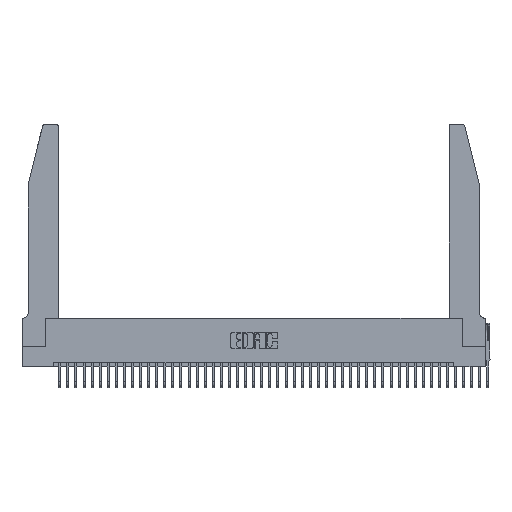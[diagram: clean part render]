
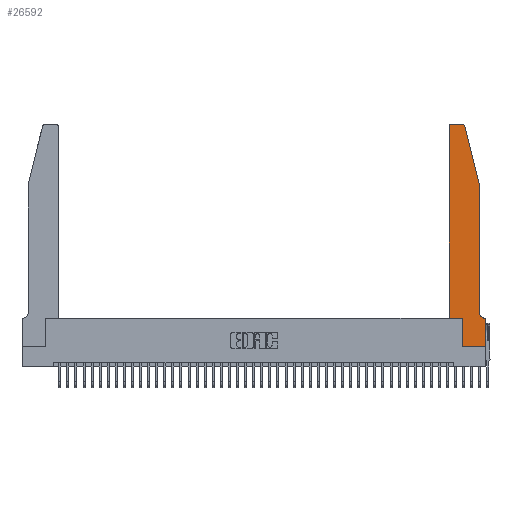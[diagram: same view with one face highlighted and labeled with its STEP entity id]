
A CAD part, top view. The second image highlights one B-rep face of the part: STEP entity #26592.
In plain terms, the highlighted face is planar.
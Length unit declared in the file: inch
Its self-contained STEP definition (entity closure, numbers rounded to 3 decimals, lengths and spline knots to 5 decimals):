
#237 = ORIENTED_EDGE ( 'NONE', *, *, #25294, .T. ) ;
#740 = LINE ( 'NONE', #4689, #40770 ) ;
#877 = CARTESIAN_POINT ( 'NONE',  ( 0.2865, 0., 0. ) ) ;
#1128 = CARTESIAN_POINT ( 'NONE',  ( 0., 0., 0. ) ) ;
#2082 = VECTOR ( 'NONE', #20227, 39.37008 ) ;
#2173 = DIRECTION ( 'NONE',  ( 1., 0., 0. ) ) ;
#3044 = ORIENTED_EDGE ( 'NONE', *, *, #37719, .F. ) ;
#4019 = EDGE_LOOP ( 'NONE', ( #30039, #237, #3044, #28536, #36588, #27299, #21938, #24894, #7005, #23495, #31857, #4577 ) ) ;
#4577 = ORIENTED_EDGE ( 'NONE', *, *, #32774, .F. ) ;
#4689 = CARTESIAN_POINT ( 'NONE',  ( 0.2605, 2.75, 0. ) ) ;
#5472 = CARTESIAN_POINT ( 'NONE',  ( 0.284, 2.72, 0. ) ) ;
#6155 = VERTEX_POINT ( 'NONE', #29059 ) ;
#6216 = CARTESIAN_POINT ( 'NONE',  ( 0., 0.35, 0. ) ) ;
#6275 = EDGE_CURVE ( 'NONE', #28637, #33616, #25479, .T. ) ;
#6299 = VECTOR ( 'NONE', #40097, 39.37008 ) ;
#6495 = AXIS2_PLACEMENT_3D ( 'NONE', #40020, #21285, #2173 ) ;
#6599 = VERTEX_POINT ( 'NONE', #21896 ) ;
#7005 = ORIENTED_EDGE ( 'NONE', *, *, #9916, .F. ) ;
#7123 = CARTESIAN_POINT ( 'NONE',  ( 0.4505, 0.35, 0. ) ) ;
#7126 = CARTESIAN_POINT ( 'NONE',  ( 0.2865, 0.35, 0. ) ) ;
#7262 = DIRECTION ( 'NONE',  ( 0., -1., 0. ) ) ;
#7534 = VERTEX_POINT ( 'NONE', #7123 ) ;
#7958 = DIRECTION ( 'NONE',  ( -1., 0., 0. ) ) ;
#8721 = DIRECTION ( 'NONE',  ( 1., 0., 0. ) ) ;
#9916 = EDGE_CURVE ( 'NONE', #24968, #28637, #20847, .T. ) ;
#10402 = EDGE_CURVE ( 'NONE', #6599, #26101, #40852, .T. ) ;
#10590 = CARTESIAN_POINT ( 'NONE',  ( 0.4205, 2.75, 0. ) ) ;
#10946 = VECTOR ( 'NONE', #12079, 39.37008 ) ;
#11057 = CARTESIAN_POINT ( 'NONE',  ( 0.0755, 2., 0. ) ) ;
#11834 = EDGE_CURVE ( 'NONE', #26124, #21214, #21745, .T. ) ;
#11879 = AXIS2_PLACEMENT_3D ( 'NONE', #5472, #27691, #8721 ) ;
#12079 = DIRECTION ( 'NONE',  ( -1., 0., 0. ) ) ;
#12393 = VECTOR ( 'NONE', #7262, 39.37008 ) ;
#12526 = EDGE_CURVE ( 'NONE', #23702, #6155, #35890, .T. ) ;
#13228 = CIRCLE ( 'NONE', #11879, 0.03 ) ;
#13244 = VECTOR ( 'NONE', #14206, 39.37008 ) ;
#13480 = CARTESIAN_POINT ( 'NONE',  ( 0.0055, 0.35, 0. ) ) ;
#13980 = CARTESIAN_POINT ( 'NONE',  ( 0.4505, 0.35, 0. ) ) ;
#14206 = DIRECTION ( 'NONE',  ( -0.239, -0.971, 0. ) ) ;
#14750 = LINE ( 'NONE', #15842, #6299 ) ;
#15842 = CARTESIAN_POINT ( 'NONE',  ( 0.4505, 0.35, 0. ) ) ;
#15997 = DIRECTION ( 'NONE',  ( 0., -1., 0. ) ) ;
#16125 = VECTOR ( 'NONE', #36067, 39.37008 ) ;
#16715 = CARTESIAN_POINT ( 'NONE',  ( 0.0055, 0.42, 0. ) ) ;
#16743 = CARTESIAN_POINT ( 'NONE',  ( 0., 0., 0. ) ) ;
#17090 = EDGE_CURVE ( 'NONE', #33616, #37558, #30803, .T. ) ;
#17521 = CARTESIAN_POINT ( 'NONE',  ( 0.284, 2.75, 0. ) ) ;
#18106 = EDGE_CURVE ( 'NONE', #26101, #24968, #19386, .T. ) ;
#19359 = AXIS2_PLACEMENT_3D ( 'NONE', #6216, #40949, #22250 ) ;
#19386 = LINE ( 'NONE', #40407, #10946 ) ;
#19905 = CARTESIAN_POINT ( 'NONE',  ( 0.25487, 2.72718, 0. ) ) ;
#19927 = DIRECTION ( 'NONE',  ( -1., 0., 0. ) ) ;
#20227 = DIRECTION ( 'NONE',  ( 1., 0., 0. ) ) ;
#20847 = LINE ( 'NONE', #16743, #12393 ) ;
#21214 = VERTEX_POINT ( 'NONE', #27109 ) ;
#21285 = DIRECTION ( 'NONE',  ( 0., 0., -1. ) ) ;
#21745 = LINE ( 'NONE', #11057, #13244 ) ;
#21896 = CARTESIAN_POINT ( 'NONE',  ( 0.0755, 0.42, 0. ) ) ;
#21938 = ORIENTED_EDGE ( 'NONE', *, *, #17090, .F. ) ;
#22250 = DIRECTION ( 'NONE',  ( 1., 0., 0. ) ) ;
#23108 = CARTESIAN_POINT ( 'NONE',  ( 0.2865, 0.35, 0. ) ) ;
#23495 = ORIENTED_EDGE ( 'NONE', *, *, #18106, .F. ) ;
#23702 = VERTEX_POINT ( 'NONE', #10590 ) ;
#24716 = VERTEX_POINT ( 'NONE', #17521 ) ;
#24833 = VECTOR ( 'NONE', #15997, 39.37008 ) ;
#24894 = ORIENTED_EDGE ( 'NONE', *, *, #6275, .F. ) ;
#24968 = VERTEX_POINT ( 'NONE', #32139 ) ;
#25294 = EDGE_CURVE ( 'NONE', #26124, #24716, #13228, .T. ) ;
#25479 = LINE ( 'NONE', #1128, #2082 ) ;
#26101 = VERTEX_POINT ( 'NONE', #13480 ) ;
#26124 = VERTEX_POINT ( 'NONE', #19905 ) ;
#26592 = ADVANCED_FACE ( 'NONE', ( #39228 ), #34565, .F. ) ;
#26753 = LINE ( 'NONE', #31739, #24833 ) ;
#27109 = CARTESIAN_POINT ( 'NONE',  ( 0.0755, 2., 0. ) ) ;
#27299 = ORIENTED_EDGE ( 'NONE', *, *, #39704, .F. ) ;
#27691 = DIRECTION ( 'NONE',  ( 0., 0., -1. ) ) ;
#28536 = ORIENTED_EDGE ( 'NONE', *, *, #12526, .T. ) ;
#28637 = VERTEX_POINT ( 'NONE', #32275 ) ;
#29059 = CARTESIAN_POINT ( 'NONE',  ( 0.4505, 2.72, 0. ) ) ;
#30039 = ORIENTED_EDGE ( 'NONE', *, *, #11834, .F. ) ;
#30803 = LINE ( 'NONE', #7126, #38141 ) ;
#31739 = CARTESIAN_POINT ( 'NONE',  ( 0.0755, 2., 0. ) ) ;
#31857 = ORIENTED_EDGE ( 'NONE', *, *, #10402, .F. ) ;
#32139 = CARTESIAN_POINT ( 'NONE',  ( 0., 0.35, 0. ) ) ;
#32275 = CARTESIAN_POINT ( 'NONE',  ( 0., 0., 0. ) ) ;
#32774 = EDGE_CURVE ( 'NONE', #21214, #6599, #26753, .T. ) ;
#32920 = LINE ( 'NONE', #13980, #16125 ) ;
#33616 = VERTEX_POINT ( 'NONE', #877 ) ;
#34565 = PLANE ( 'NONE',  #19359 ) ;
#35591 = DIRECTION ( 'NONE',  ( 0., 1., 0. ) ) ;
#35890 = CIRCLE ( 'NONE', #6495, 0.03 ) ;
#36067 = DIRECTION ( 'NONE',  ( 1., 0., 0. ) ) ;
#36588 = ORIENTED_EDGE ( 'NONE', *, *, #38040, .F. ) ;
#37402 = AXIS2_PLACEMENT_3D ( 'NONE', #16715, #38704, #19927 ) ;
#37558 = VERTEX_POINT ( 'NONE', #23108 ) ;
#37719 = EDGE_CURVE ( 'NONE', #23702, #24716, #740, .T. ) ;
#38040 = EDGE_CURVE ( 'NONE', #7534, #6155, #14750, .T. ) ;
#38141 = VECTOR ( 'NONE', #35591, 39.37008 ) ;
#38704 = DIRECTION ( 'NONE',  ( 0., 0., -1. ) ) ;
#39228 = FACE_OUTER_BOUND ( 'NONE', #4019, .T. ) ;
#39704 = EDGE_CURVE ( 'NONE', #37558, #7534, #32920, .T. ) ;
#40020 = CARTESIAN_POINT ( 'NONE',  ( 0.4205, 2.72, 0. ) ) ;
#40097 = DIRECTION ( 'NONE',  ( 0., 1., 0. ) ) ;
#40407 = CARTESIAN_POINT ( 'NONE',  ( 0.0755, 0.35, 0. ) ) ;
#40770 = VECTOR ( 'NONE', #7958, 39.37008 ) ;
#40852 = CIRCLE ( 'NONE', #37402, 0.07 ) ;
#40949 = DIRECTION ( 'NONE',  ( 0., 0., 1. ) ) ;
